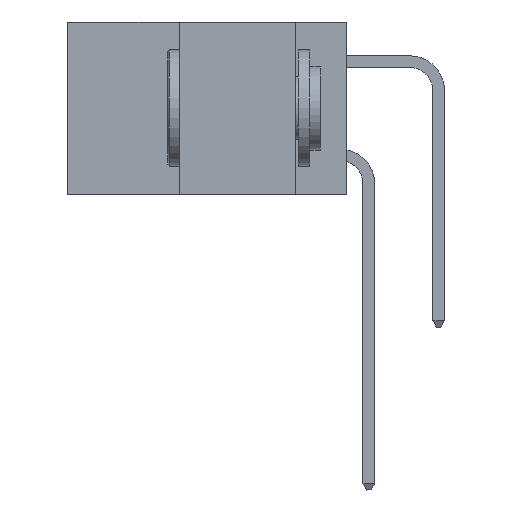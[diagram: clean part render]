
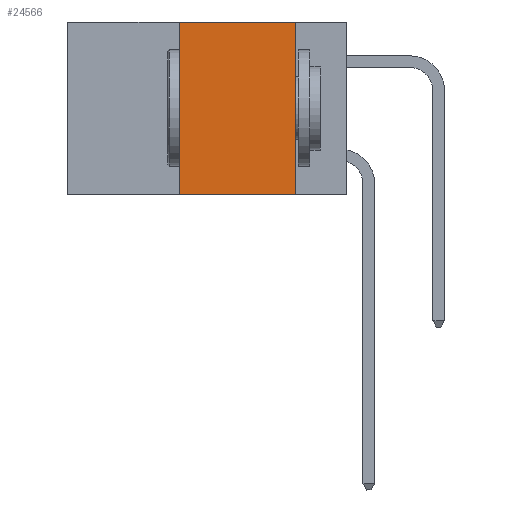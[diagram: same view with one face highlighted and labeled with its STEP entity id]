
A CAD part, left-side view. The second image highlights one B-rep face of the part: STEP entity #24566.
In plain terms, the highlighted planar face has unit normal (-1, 0, 0).
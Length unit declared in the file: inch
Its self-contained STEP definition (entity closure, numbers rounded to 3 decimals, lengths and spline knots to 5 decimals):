
#296 = DIRECTION ( 'NONE',  ( 1., 0., 0. ) ) ;
#4727 = CARTESIAN_POINT ( 'NONE',  ( 0., 0.36, 0. ) ) ;
#5817 = ORIENTED_EDGE ( 'NONE', *, *, #8982, .T. ) ;
#6845 = CARTESIAN_POINT ( 'NONE',  ( 0., 0.6, 0. ) ) ;
#7647 = VECTOR ( 'NONE', #10075, 39.37008 ) ;
#8320 = CARTESIAN_POINT ( 'NONE',  ( 0., 0.36, -0.37 ) ) ;
#8488 = EDGE_CURVE ( 'NONE', #10573, #22492, #14214, .T. ) ;
#8828 = DIRECTION ( 'NONE',  ( 0., -1., 0. ) ) ;
#8907 = VECTOR ( 'NONE', #10643, 39.37008 ) ;
#8982 = EDGE_CURVE ( 'NONE', #10554, #22492, #12963, .T. ) ;
#9868 = ORIENTED_EDGE ( 'NONE', *, *, #8488, .F. ) ;
#10075 = DIRECTION ( 'NONE',  ( 0., -1., 0. ) ) ;
#10512 = ORIENTED_EDGE ( 'NONE', *, *, #12651, .F. ) ;
#10554 = VERTEX_POINT ( 'NONE', #8320 ) ;
#10573 = VERTEX_POINT ( 'NONE', #24202 ) ;
#10643 = DIRECTION ( 'NONE',  ( 0., 0., -1. ) ) ;
#10771 = DIRECTION ( 'NONE',  ( 0., 0., 1. ) ) ;
#12332 = PLANE ( 'NONE',  #21242 ) ;
#12651 = EDGE_CURVE ( 'NONE', #12720, #10573, #15645, .T. ) ;
#12720 = VERTEX_POINT ( 'NONE', #15007 ) ;
#12963 = LINE ( 'NONE', #16014, #7647 ) ;
#13382 = CARTESIAN_POINT ( 'NONE',  ( 0., 0.11, -0.37 ) ) ;
#13537 = VECTOR ( 'NONE', #10771, 39.37008 ) ;
#14207 = EDGE_LOOP ( 'NONE', ( #9868, #10512, #21061, #5817 ) ) ;
#14214 = LINE ( 'NONE', #24337, #8907 ) ;
#14305 = DIRECTION ( 'NONE',  ( 0., 0., -1. ) ) ;
#15007 = CARTESIAN_POINT ( 'NONE',  ( 0., 0.36, 0. ) ) ;
#15645 = LINE ( 'NONE', #6845, #25418 ) ;
#16014 = CARTESIAN_POINT ( 'NONE',  ( 0., 0.6, -0.37 ) ) ;
#18243 = CARTESIAN_POINT ( 'NONE',  ( 0., 0.6, 0. ) ) ;
#19435 = LINE ( 'NONE', #4727, #13537 ) ;
#21061 = ORIENTED_EDGE ( 'NONE', *, *, #22259, .F. ) ;
#21242 = AXIS2_PLACEMENT_3D ( 'NONE', #18243, #296, #14305 ) ;
#21445 = FACE_OUTER_BOUND ( 'NONE', #14207, .T. ) ;
#22259 = EDGE_CURVE ( 'NONE', #10554, #12720, #19435, .T. ) ;
#22492 = VERTEX_POINT ( 'NONE', #13382 ) ;
#24202 = CARTESIAN_POINT ( 'NONE',  ( 0., 0.11, 0. ) ) ;
#24337 = CARTESIAN_POINT ( 'NONE',  ( 0., 0.11, 0. ) ) ;
#24566 = ADVANCED_FACE ( 'NONE', ( #21445 ), #12332, .F. ) ;
#25418 = VECTOR ( 'NONE', #8828, 39.37008 ) ;
